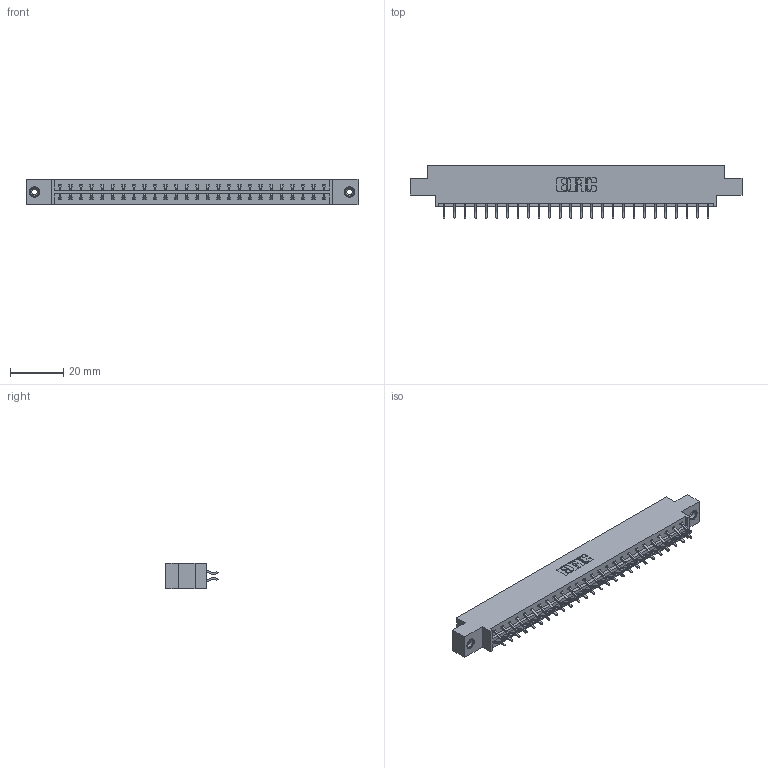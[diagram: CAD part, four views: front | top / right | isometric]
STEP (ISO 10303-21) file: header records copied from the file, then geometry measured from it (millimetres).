
FILE_DESCRIPTION (( 'STEP AP203' ), '1' );
FILE_NAME ('833-052-556-808.STEP', '2020-06-04T19:50:34', ( '' ), ( '' ), 'SwSTEP 2.0', 'SolidWorks 2020', '' );
FILE_SCHEMA (( 'CONFIG_CONTROL_DESIGN' ));
Length unit declared in the file: inch
Products named in the file (4): 345-250-001_345-250-003-102; 833-052-556-808; 345-292-001_556 Tail; 833 Part_Offset - .156 Dia - TI
Assembly tree (55 placements, depth 2):
  833-052-556-808
    833 Part_Offset - .156 Dia - TI
    345-292-001_556 Tail  x52
    345-250-001_345-250-003-102  x2
Bounding box: 124.56 x 19.57 x 9.4 mm (x, y, z)
Volume: 12331 mm3; surface area: 14597.7 mm2
Topology: 55 solids, 55 shells, 3194 faces, 9455 edges, 6226 vertices
Faces by surface type: plane 2186, cylinder 992, cone 12, torus 4
Entity records: 20334 total; most frequent: CARTESIAN_POINT 3389, ORIENTED_EDGE 3306, DIRECTION 2943, EDGE_CURVE 1653, LINE 1497, VECTOR 1497, VERTEX_POINT 1096, AXIS2_PLACEMENT_3D 723
